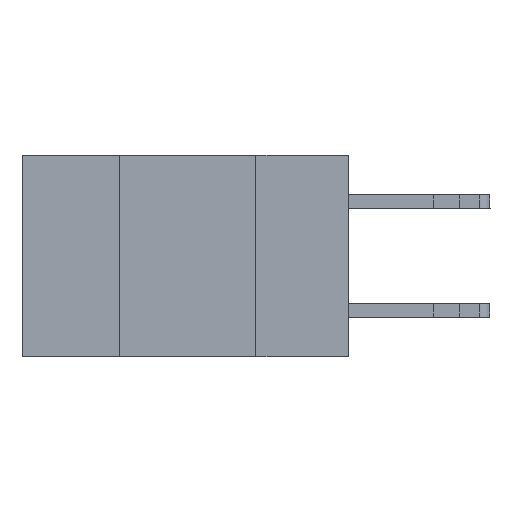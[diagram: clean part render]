
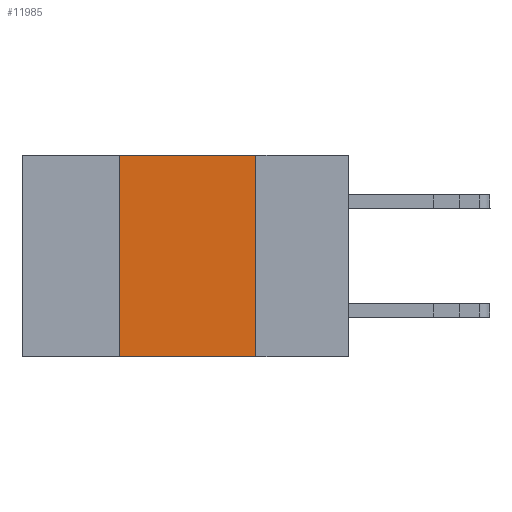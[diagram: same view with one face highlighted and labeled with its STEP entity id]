
A CAD part, left-side view. The second image highlights one B-rep face of the part: STEP entity #11985.
In plain terms, the highlighted planar face has unit normal (-1, 0, 0).
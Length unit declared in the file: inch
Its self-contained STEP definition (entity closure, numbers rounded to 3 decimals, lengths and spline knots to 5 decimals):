
#402 = CARTESIAN_POINT ( 'NONE',  ( 0., 0.6, 0. ) ) ;
#1365 = CARTESIAN_POINT ( 'NONE',  ( 0., 0.6, -0.37 ) ) ;
#1552 = ORIENTED_EDGE ( 'NONE', *, *, #9223, .T. ) ;
#2034 = CARTESIAN_POINT ( 'NONE',  ( 0., 0.17, 0. ) ) ;
#2267 = CARTESIAN_POINT ( 'NONE',  ( 0., 0.17, -0.37 ) ) ;
#2474 = EDGE_CURVE ( 'NONE', #9508, #5715, #7800, .T. ) ;
#2643 = AXIS2_PLACEMENT_3D ( 'NONE', #402, #4812, #3725 ) ;
#3623 = VERTEX_POINT ( 'NONE', #2267 ) ;
#3725 = DIRECTION ( 'NONE',  ( 0., 0., -1. ) ) ;
#3965 = VECTOR ( 'NONE', #6721, 39.37008 ) ;
#4051 = VERTEX_POINT ( 'NONE', #2034 ) ;
#4197 = CARTESIAN_POINT ( 'NONE',  ( 0., 0.17, -0.37 ) ) ;
#4812 = DIRECTION ( 'NONE',  ( 1., 0., 0. ) ) ;
#5059 = EDGE_CURVE ( 'NONE', #4051, #3623, #11854, .T. ) ;
#5715 = VERTEX_POINT ( 'NONE', #14128 ) ;
#6508 = VECTOR ( 'NONE', #8747, 39.37008 ) ;
#6721 = DIRECTION ( 'NONE',  ( 0., 0., 1. ) ) ;
#6955 = VECTOR ( 'NONE', #9074, 39.37008 ) ;
#7657 = CARTESIAN_POINT ( 'NONE',  ( 0., 0.6, 0. ) ) ;
#7800 = LINE ( 'NONE', #12205, #3965 ) ;
#8747 = DIRECTION ( 'NONE',  ( 0., 0., -1. ) ) ;
#8888 = LINE ( 'NONE', #7657, #12081 ) ;
#9074 = DIRECTION ( 'NONE',  ( 0., -1., 0. ) ) ;
#9223 = EDGE_CURVE ( 'NONE', #9508, #3623, #10026, .T. ) ;
#9508 = VERTEX_POINT ( 'NONE', #10855 ) ;
#10026 = LINE ( 'NONE', #1365, #6955 ) ;
#10032 = FACE_OUTER_BOUND ( 'NONE', #11643, .T. ) ;
#10128 = DIRECTION ( 'NONE',  ( 0., -1., 0. ) ) ;
#10855 = CARTESIAN_POINT ( 'NONE',  ( 0., 0.42, -0.37 ) ) ;
#11371 = PLANE ( 'NONE',  #2643 ) ;
#11466 = ORIENTED_EDGE ( 'NONE', *, *, #2474, .F. ) ;
#11643 = EDGE_LOOP ( 'NONE', ( #12717, #13389, #11466, #1552 ) ) ;
#11854 = LINE ( 'NONE', #4197, #6508 ) ;
#11985 = ADVANCED_FACE ( 'NONE', ( #10032 ), #11371, .F. ) ;
#12081 = VECTOR ( 'NONE', #10128, 39.37008 ) ;
#12205 = CARTESIAN_POINT ( 'NONE',  ( 0., 0.42, -0.37 ) ) ;
#12717 = ORIENTED_EDGE ( 'NONE', *, *, #5059, .F. ) ;
#13389 = ORIENTED_EDGE ( 'NONE', *, *, #14022, .F. ) ;
#14022 = EDGE_CURVE ( 'NONE', #5715, #4051, #8888, .T. ) ;
#14128 = CARTESIAN_POINT ( 'NONE',  ( 0., 0.42, 0. ) ) ;
